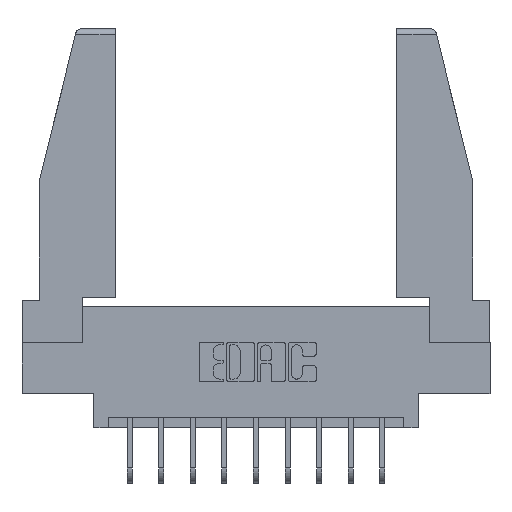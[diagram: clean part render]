
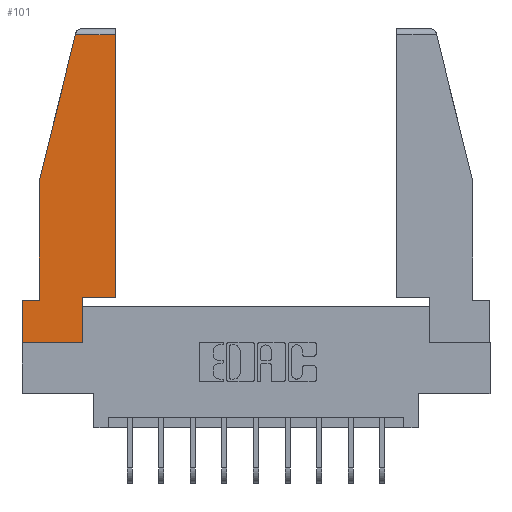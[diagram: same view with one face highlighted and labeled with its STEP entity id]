
A CAD part, top view. The second image highlights one B-rep face of the part: STEP entity #101.
In plain terms, the highlighted planar face has unit normal (0, 0, 1).
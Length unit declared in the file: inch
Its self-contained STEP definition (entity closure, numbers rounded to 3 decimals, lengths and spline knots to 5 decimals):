
#70 = LINE ( 'NONE', #7811, #13662 ) ;
#101 = ADVANCED_FACE ( 'NONE', ( #9846 ), #12405, .T. ) ;
#353 = ORIENTED_EDGE ( 'NONE', *, *, #8888, .T. ) ;
#419 = VERTEX_POINT ( 'NONE', #8067 ) ;
#441 = CARTESIAN_POINT ( 'NONE',  ( 0.271, 1.55, 0. ) ) ;
#449 = ORIENTED_EDGE ( 'NONE', *, *, #8655, .T. ) ;
#647 = VECTOR ( 'NONE', #14870, 39.37008 ) ;
#1224 = VECTOR ( 'NONE', #2049, 39.37008 ) ;
#1367 = VECTOR ( 'NONE', #13751, 39.37008 ) ;
#1406 = LINE ( 'NONE', #7058, #1224 ) ;
#1450 = CARTESIAN_POINT ( 'NONE',  ( 0.297, 0.223, 0. ) ) ;
#1834 = DIRECTION ( 'NONE',  ( 0., 1., 0. ) ) ;
#1857 = VECTOR ( 'NONE', #3275, 39.37008 ) ;
#2018 = ORIENTED_EDGE ( 'NONE', *, *, #13143, .T. ) ;
#2024 = ORIENTED_EDGE ( 'NONE', *, *, #7835, .T. ) ;
#2049 = DIRECTION ( 'NONE',  ( -1., 0., 0. ) ) ;
#2186 = VERTEX_POINT ( 'NONE', #11586 ) ;
#2285 = LINE ( 'NONE', #6583, #4503 ) ;
#2321 = CARTESIAN_POINT ( 'NONE',  ( 0.086, 0.21, 0. ) ) ;
#2582 = ORIENTED_EDGE ( 'NONE', *, *, #9722, .T. ) ;
#2607 = DIRECTION ( 'NONE',  ( 0., 0., 1. ) ) ;
#2659 = LINE ( 'NONE', #2883, #5615 ) ;
#2883 = CARTESIAN_POINT ( 'NONE',  ( 0.461, 0.223, 0. ) ) ;
#3275 = DIRECTION ( 'NONE',  ( 1., 0., 0. ) ) ;
#4450 = EDGE_LOOP ( 'NONE', ( #2018, #13723, #8662, #449, #2024, #2582, #5165, #353, #4974 ) ) ;
#4466 = AXIS2_PLACEMENT_3D ( 'NONE', #6126, #2607, #7356 ) ;
#4503 = VECTOR ( 'NONE', #10199, 39.37008 ) ;
#4974 = ORIENTED_EDGE ( 'NONE', *, *, #13631, .T. ) ;
#5151 = CARTESIAN_POINT ( 'NONE',  ( 0.461, 0.223, 0. ) ) ;
#5165 = ORIENTED_EDGE ( 'NONE', *, *, #7731, .T. ) ;
#5450 = VECTOR ( 'NONE', #9214, 39.37008 ) ;
#5591 = DIRECTION ( 'NONE',  ( -1., 0., 0. ) ) ;
#5615 = VECTOR ( 'NONE', #1834, 39.37008 ) ;
#5878 = LINE ( 'NONE', #12510, #14636 ) ;
#6126 = CARTESIAN_POINT ( 'NONE',  ( 0., 0., 0. ) ) ;
#6583 = CARTESIAN_POINT ( 'NONE',  ( 0., 0.21, 0. ) ) ;
#7058 = CARTESIAN_POINT ( 'NONE',  ( 0., 1.52, 0. ) ) ;
#7144 = CARTESIAN_POINT ( 'NONE',  ( 0.086, 0.8, 0. ) ) ;
#7201 = VERTEX_POINT ( 'NONE', #11354 ) ;
#7214 = EDGE_CURVE ( 'NONE', #10529, #15413, #10273, .T. ) ;
#7356 = DIRECTION ( 'NONE',  ( 1., 0., 0. ) ) ;
#7731 = EDGE_CURVE ( 'NONE', #7201, #12632, #5878, .T. ) ;
#7811 = CARTESIAN_POINT ( 'NONE',  ( 0., 0.21, 0. ) ) ;
#7835 = EDGE_CURVE ( 'NONE', #10018, #419, #70, .T. ) ;
#8040 = CARTESIAN_POINT ( 'NONE',  ( 0.297, 0., 0. ) ) ;
#8067 = CARTESIAN_POINT ( 'NONE',  ( 0., 0.21, 0. ) ) ;
#8655 = EDGE_CURVE ( 'NONE', #15413, #10018, #14215, .T. ) ;
#8662 = ORIENTED_EDGE ( 'NONE', *, *, #7214, .T. ) ;
#8888 = EDGE_CURVE ( 'NONE', #12632, #15306, #12669, .T. ) ;
#9214 = DIRECTION ( 'NONE',  ( 0., 1., 0. ) ) ;
#9279 = CARTESIAN_POINT ( 'NONE',  ( 0.297, 0.223, 0. ) ) ;
#9722 = EDGE_CURVE ( 'NONE', #419, #7201, #2285, .T. ) ;
#9779 = LINE ( 'NONE', #9279, #1857 ) ;
#9846 = FACE_OUTER_BOUND ( 'NONE', #4450, .T. ) ;
#10018 = VERTEX_POINT ( 'NONE', #2321 ) ;
#10111 = DIRECTION ( 'NONE',  ( 1., 0., 0. ) ) ;
#10199 = DIRECTION ( 'NONE',  ( 0., -1., 0. ) ) ;
#10273 = LINE ( 'NONE', #441, #647 ) ;
#10529 = VERTEX_POINT ( 'NONE', #14307 ) ;
#11214 = CARTESIAN_POINT ( 'NONE',  ( 0.086, 0.8, 0. ) ) ;
#11279 = CARTESIAN_POINT ( 'NONE',  ( 0.297, 0., 0. ) ) ;
#11354 = CARTESIAN_POINT ( 'NONE',  ( 0., 0., 0. ) ) ;
#11586 = CARTESIAN_POINT ( 'NONE',  ( 0.461, 1.52, 0. ) ) ;
#12405 = PLANE ( 'NONE',  #4466 ) ;
#12510 = CARTESIAN_POINT ( 'NONE',  ( 0., 0., 0. ) ) ;
#12632 = VERTEX_POINT ( 'NONE', #11279 ) ;
#12669 = LINE ( 'NONE', #8040, #5450 ) ;
#13143 = EDGE_CURVE ( 'NONE', #15205, #2186, #2659, .T. ) ;
#13631 = EDGE_CURVE ( 'NONE', #15306, #15205, #9779, .T. ) ;
#13662 = VECTOR ( 'NONE', #5591, 39.37008 ) ;
#13723 = ORIENTED_EDGE ( 'NONE', *, *, #14851, .T. ) ;
#13751 = DIRECTION ( 'NONE',  ( 0., -1., 0. ) ) ;
#14215 = LINE ( 'NONE', #11214, #1367 ) ;
#14307 = CARTESIAN_POINT ( 'NONE',  ( 0.2636, 1.52, 0. ) ) ;
#14636 = VECTOR ( 'NONE', #10111, 39.37008 ) ;
#14851 = EDGE_CURVE ( 'NONE', #2186, #10529, #1406, .T. ) ;
#14870 = DIRECTION ( 'NONE',  ( -0.239, -0.971, 0. ) ) ;
#15205 = VERTEX_POINT ( 'NONE', #5151 ) ;
#15306 = VERTEX_POINT ( 'NONE', #1450 ) ;
#15413 = VERTEX_POINT ( 'NONE', #7144 ) ;
